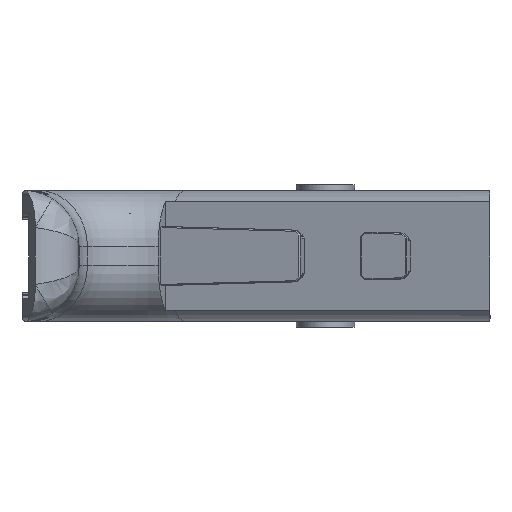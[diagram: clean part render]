
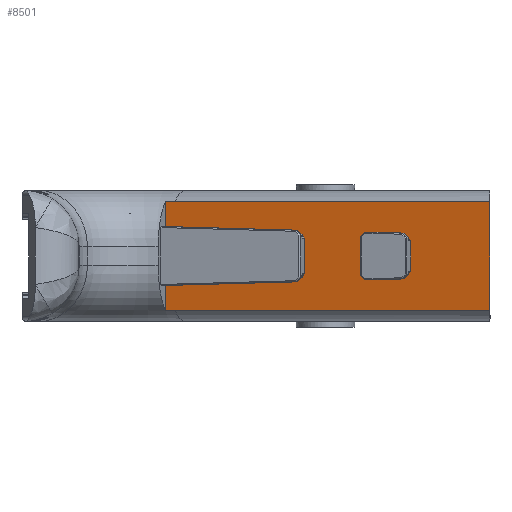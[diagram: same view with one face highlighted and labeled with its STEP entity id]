
A CAD part, left-side view. The second image highlights one B-rep face of the part: STEP entity #8501.
In plain terms, the highlighted planar face has unit normal (-0.951, 0.309, 0).
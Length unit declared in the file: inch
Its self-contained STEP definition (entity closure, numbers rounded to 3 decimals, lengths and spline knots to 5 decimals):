
#502=FACE_BOUND('',#1396,.T.);
#588=PLANE('',#9039);
#901=FACE_OUTER_BOUND('',#1395,.T.);
#1395=EDGE_LOOP('',(#6215,#6216,#6217,#6218,#6219,#6220,#6221,#6222,#6223,
#6224,#6225,#6226));
#1396=EDGE_LOOP('',(#6227,#6228,#6229,#6230,#6231,#6232,#6233,#6234,#6235));
#1954=LINE('',#24706,#2847);
#1972=LINE('',#24744,#2865);
#1980=LINE('',#24761,#2873);
#1985=LINE('',#24770,#2878);
#1987=LINE('',#24773,#2880);
#1989=LINE('',#24778,#2882);
#1991=LINE('',#24782,#2884);
#1993=LINE('',#24785,#2886);
#1995=LINE('',#24789,#2888);
#1996=LINE('',#24791,#2889);
#2002=LINE('',#24804,#2895);
#2004=LINE('',#24808,#2897);
#2005=LINE('',#24811,#2898);
#2007=LINE('',#24815,#2900);
#2008=LINE('',#24825,#2901);
#2009=LINE('',#24827,#2902);
#2010=LINE('',#24829,#2903);
#2011=LINE('',#24839,#2904);
#2012=LINE('',#24840,#2905);
#2847=VECTOR('',#9966,0.3937);
#2865=VECTOR('',#10002,0.3937);
#2873=VECTOR('',#10016,0.3937);
#2878=VECTOR('',#10025,0.3937);
#2880=VECTOR('',#10029,0.3937);
#2882=VECTOR('',#10033,0.3937);
#2884=VECTOR('',#10037,0.3937);
#2886=VECTOR('',#10041,0.3937);
#2888=VECTOR('',#10045,0.3937);
#2889=VECTOR('',#10048,0.3937);
#2895=VECTOR('',#10064,0.3937);
#2897=VECTOR('',#10068,0.3937);
#2898=VECTOR('',#10071,0.3937);
#2900=VECTOR('',#10075,0.3937);
#2901=VECTOR('',#10076,0.3937);
#2902=VECTOR('',#10077,0.3937);
#2903=VECTOR('',#10078,0.3937);
#2904=VECTOR('',#10079,0.3937);
#2905=VECTOR('',#10080,0.3937);
#3611=B_SPLINE_CURVE_WITH_KNOTS('',3,(#24817,#24818,#24819,#24820,#24821,
#24822,#24823),.UNSPECIFIED.,.F.,.F.,(4,3,4),(0.,0.1181,0.21548),
 .UNSPECIFIED.);
#3612=B_SPLINE_CURVE_WITH_KNOTS('',3,(#24831,#24832,#24833,#24834,#24835,
#24836,#24837),.UNSPECIFIED.,.F.,.F.,(4,3,4),(-0.21548,-0.1181,
0.),.UNSPECIFIED.);
#3836=VERTEX_POINT('',#24703);
#3837=VERTEX_POINT('',#24705);
#3847=VERTEX_POINT('',#24741);
#3848=VERTEX_POINT('',#24743);
#3853=VERTEX_POINT('',#24758);
#3854=VERTEX_POINT('',#24760);
#3856=VERTEX_POINT('',#24769);
#3857=VERTEX_POINT('',#24775);
#3858=VERTEX_POINT('',#24777);
#3859=VERTEX_POINT('',#24781);
#3860=VERTEX_POINT('',#24787);
#3862=VERTEX_POINT('',#24802);
#3863=VERTEX_POINT('',#24806);
#3864=VERTEX_POINT('',#24810);
#3865=VERTEX_POINT('',#24814);
#3866=VERTEX_POINT('',#24816);
#3867=VERTEX_POINT('',#24824);
#3868=VERTEX_POINT('',#24826);
#3869=VERTEX_POINT('',#24828);
#3870=VERTEX_POINT('',#24830);
#3871=VERTEX_POINT('',#24838);
#4707=EDGE_CURVE('',#3837,#3836,#1954,.T.);
#4725=EDGE_CURVE('',#3847,#3848,#1972,.T.);
#4733=EDGE_CURVE('',#3853,#3854,#1980,.F.);
#4738=EDGE_CURVE('',#3837,#3856,#1985,.F.);
#4740=EDGE_CURVE('',#3853,#3856,#1987,.T.);
#4742=EDGE_CURVE('',#3857,#3858,#1989,.F.);
#4744=EDGE_CURVE('',#3859,#3858,#1991,.T.);
#4746=EDGE_CURVE('',#3857,#3854,#1993,.T.);
#4748=EDGE_CURVE('',#3860,#3836,#1995,.F.);
#4749=EDGE_CURVE('',#3859,#3860,#1996,.F.);
#4755=EDGE_CURVE('',#3862,#3847,#2002,.F.);
#4757=EDGE_CURVE('',#3862,#3863,#2004,.T.);
#4758=EDGE_CURVE('',#3848,#3864,#2005,.F.);
#4760=EDGE_CURVE('',#3865,#3863,#2007,.T.);
#4761=EDGE_CURVE('',#3866,#3865,#3611,.T.);
#4762=EDGE_CURVE('',#3867,#3866,#2008,.T.);
#4763=EDGE_CURVE('',#3868,#3867,#2009,.T.);
#4764=EDGE_CURVE('',#3869,#3868,#2010,.T.);
#4765=EDGE_CURVE('',#3870,#3869,#3612,.T.);
#4766=EDGE_CURVE('',#3871,#3870,#2011,.T.);
#4767=EDGE_CURVE('',#3871,#3864,#2012,.T.);
#6215=ORIENTED_EDGE('',*,*,#4757,.T.);
#6216=ORIENTED_EDGE('',*,*,#4760,.F.);
#6217=ORIENTED_EDGE('',*,*,#4761,.F.);
#6218=ORIENTED_EDGE('',*,*,#4762,.F.);
#6219=ORIENTED_EDGE('',*,*,#4763,.F.);
#6220=ORIENTED_EDGE('',*,*,#4764,.F.);
#6221=ORIENTED_EDGE('',*,*,#4765,.F.);
#6222=ORIENTED_EDGE('',*,*,#4766,.F.);
#6223=ORIENTED_EDGE('',*,*,#4767,.T.);
#6224=ORIENTED_EDGE('',*,*,#4758,.F.);
#6225=ORIENTED_EDGE('',*,*,#4725,.F.);
#6226=ORIENTED_EDGE('',*,*,#4755,.F.);
#6227=ORIENTED_EDGE('',*,*,#4707,.T.);
#6228=ORIENTED_EDGE('',*,*,#4748,.F.);
#6229=ORIENTED_EDGE('',*,*,#4749,.F.);
#6230=ORIENTED_EDGE('',*,*,#4744,.T.);
#6231=ORIENTED_EDGE('',*,*,#4742,.F.);
#6232=ORIENTED_EDGE('',*,*,#4746,.T.);
#6233=ORIENTED_EDGE('',*,*,#4733,.F.);
#6234=ORIENTED_EDGE('',*,*,#4740,.T.);
#6235=ORIENTED_EDGE('',*,*,#4738,.F.);
#8501=ADVANCED_FACE('',(#901,#502),#588,.T.);
#9039=AXIS2_PLACEMENT_3D('',#24813,#10073,#10074);
#9966=DIRECTION('',(0.,0.,1.));
#10002=DIRECTION('',(0.,0.,1.));
#10016=DIRECTION('',(0.216,0.664,-0.716));
#10025=DIRECTION('',(0.221,0.681,0.698));
#10029=DIRECTION('',(0.309,0.951,-0.026));
#10033=DIRECTION('',(-0.216,-0.664,-0.716));
#10037=DIRECTION('',(-0.309,-0.951,-0.026));
#10041=DIRECTION('',(0.,0.,-1.));
#10045=DIRECTION('',(-0.12,-0.37,0.921));
#10048=DIRECTION('',(-0.221,-0.681,0.698));
#10064=DIRECTION('',(0.216,0.664,-0.716));
#10068=DIRECTION('',(0.309,0.951,-0.026));
#10071=DIRECTION('',(-0.216,-0.664,-0.716));
#10073=DIRECTION('center_axis',(-0.951,0.309,0.));
#10074=DIRECTION('ref_axis',(0.,0.,
1.));
#10075=DIRECTION('',(0.,0.,1.));
#10076=DIRECTION('',(0.309,0.951,0.));
#10077=DIRECTION('',(0.,0.,-1.));
#10078=DIRECTION('',(-0.309,-0.951,0.));
#10079=DIRECTION('',(0.,0.,1.));
#10080=DIRECTION('',(-0.309,-0.951,-0.026));
#24703=CARTESIAN_POINT('',(-2.89621,-0.88381,-0.63519));
#24705=CARTESIAN_POINT('',(-2.89621,-0.88381,-0.91008));
#24706=CARTESIAN_POINT('',(-2.89621,-0.88381,-0.76772));
#24741=CARTESIAN_POINT('',(-2.72625,-0.36073,-0.92448));
#24743=CARTESIAN_POINT('',(-2.72625,-0.36073,-0.61095));
#24744=CARTESIAN_POINT('',(-2.72625,-0.36073,-0.91535));
#24758=CARTESIAN_POINT('',(-3.02469,-1.27924,-0.90904));
#24760=CARTESIAN_POINT('',(-3.02773,-1.2886,-0.89894));
#24761=CARTESIAN_POINT('',(-2.99079,-1.1749,-1.02165));
#24769=CARTESIAN_POINT('',(-2.89925,-0.89317,-0.91967));
#24770=CARTESIAN_POINT('',(-2.87091,-0.80595,-0.83033));
#24773=CARTESIAN_POINT('',(-3.04691,-1.34763,-0.90715));
#24775=CARTESIAN_POINT('',(-3.02773,-1.2886,-0.6365));
#24777=CARTESIAN_POINT('',(-3.02469,-1.27924,-0.6264));
#24778=CARTESIAN_POINT('',(-2.99079,-1.1749,-0.51378));
#24781=CARTESIAN_POINT('',(-2.89925,-0.89317,-0.61577));
#24782=CARTESIAN_POINT('',(-3.04691,-1.34763,-0.62828));
#24785=CARTESIAN_POINT('',(-3.02773,-1.2886,-0.89897));
#24787=CARTESIAN_POINT('',(-2.89839,-0.89052,-0.61848));
#24789=CARTESIAN_POINT('',(-2.88498,-0.84927,-0.72129));
#24791=CARTESIAN_POINT('',(-2.87091,-0.80595,-0.7051));
#24802=CARTESIAN_POINT('',(-2.72321,-0.35137,-0.93458));
#24804=CARTESIAN_POINT('',(-2.76468,-0.479,-0.79683));
#24806=CARTESIAN_POINT('',(-2.33244,0.85128,-0.9677));
#24808=CARTESIAN_POINT('',(-3.04691,-1.34763,-0.90715));
#24810=CARTESIAN_POINT('',(-2.72321,-0.35137,-0.60085));
#24811=CARTESIAN_POINT('',(-2.76468,-0.479,-0.73861));
#24813=CARTESIAN_POINT('Origin',(-2.83749,-0.7031,-0.76772));
#24814=CARTESIAN_POINT('',(-2.33244,0.85128,-1.24594));
#24815=CARTESIAN_POINT('',(-2.33244,0.85128,-1.03022));
#24816=CARTESIAN_POINT('',(-2.35921,0.76891,-1.2425));
#24817=CARTESIAN_POINT('Ctrl Pts',(-2.35921,0.76891,
-1.2425));
#24818=CARTESIAN_POINT('Ctrl Pts',(-2.35442,0.78365,
-1.2425));
#24819=CARTESIAN_POINT('Ctrl Pts',(-2.34954,0.79864,
-1.24284));
#24820=CARTESIAN_POINT('Ctrl Pts',(-2.34461,0.81384,
-1.24353));
#24821=CARTESIAN_POINT('Ctrl Pts',(-2.34054,0.82637,
-1.24411));
#24822=CARTESIAN_POINT('Ctrl Pts',(-2.33649,0.83883,
-1.24492));
#24823=CARTESIAN_POINT('Ctrl Pts',(-2.33244,0.85128,-1.24594));
#24824=CARTESIAN_POINT('',(-3.25158,-1.97753,-1.2425));
#24825=CARTESIAN_POINT('',(-2.19691,1.2684,-1.2425));
#24826=CARTESIAN_POINT('',(-3.25158,-1.97753,-0.29293));
#24827=CARTESIAN_POINT('',(-3.25158,-1.97753,-0.38386));
#24828=CARTESIAN_POINT('',(-2.35921,0.76891,-0.29293));
#24829=CARTESIAN_POINT('',(-2.69056,-0.25088,-0.29293));
#24830=CARTESIAN_POINT('',(-2.33244,0.85128,-0.28949));
#24831=CARTESIAN_POINT('Ctrl Pts',(-2.33244,0.85128,-0.28949));
#24832=CARTESIAN_POINT('Ctrl Pts',(-2.33649,0.83883,
-0.29052));
#24833=CARTESIAN_POINT('Ctrl Pts',(-2.34054,0.82637,
-0.29132));
#24834=CARTESIAN_POINT('Ctrl Pts',(-2.34461,0.81384,
-0.2919));
#24835=CARTESIAN_POINT('Ctrl Pts',(-2.34954,0.79864,
-0.29259));
#24836=CARTESIAN_POINT('Ctrl Pts',(-2.35442,0.78365,
-0.29293));
#24837=CARTESIAN_POINT('Ctrl Pts',(-2.35921,0.76891,
-0.29293));
#24838=CARTESIAN_POINT('',(-2.33244,0.85128,-0.56774));
#24839=CARTESIAN_POINT('',(-2.33244,0.85128,-0.76772));
#24840=CARTESIAN_POINT('',(-3.04691,-1.34763,-0.62828));
